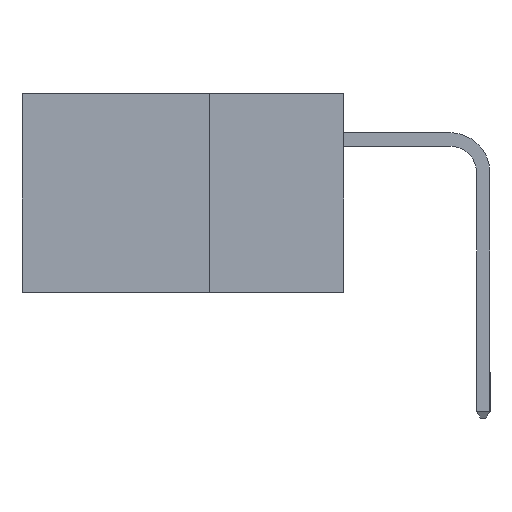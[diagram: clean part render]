
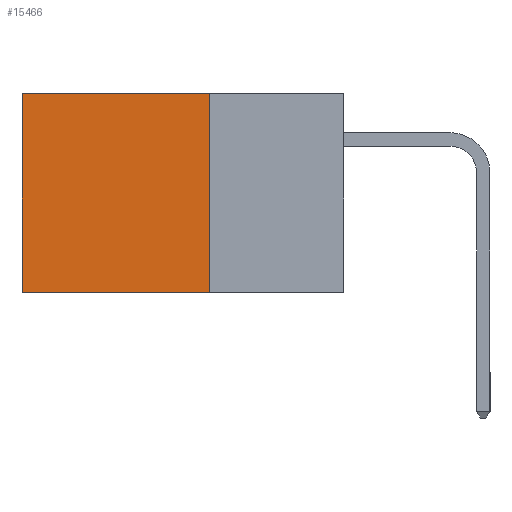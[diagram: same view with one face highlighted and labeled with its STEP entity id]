
A CAD part, left-side view. The second image highlights one B-rep face of the part: STEP entity #15466.
In plain terms, the highlighted planar face has unit normal (-1, 0, 0).
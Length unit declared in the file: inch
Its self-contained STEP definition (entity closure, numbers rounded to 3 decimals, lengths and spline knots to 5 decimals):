
#284 = DIRECTION ( 'NONE',  ( 1., 0., 0. ) ) ;
#853 = DIRECTION ( 'NONE',  ( 0., 1., 0. ) ) ;
#2207 = CARTESIAN_POINT ( 'NONE',  ( 0.2615, 0.6, -0.37 ) ) ;
#4711 = CARTESIAN_POINT ( 'NONE',  ( 0.2615, 0.25, -0.37 ) ) ;
#6311 = LINE ( 'NONE', #13989, #12401 ) ;
#6320 = CARTESIAN_POINT ( 'NONE',  ( 0.2615, 0.6, 0. ) ) ;
#6404 = AXIS2_PLACEMENT_3D ( 'NONE', #8105, #284, #21174 ) ;
#6442 = DIRECTION ( 'NONE',  ( 0., 0., -1. ) ) ;
#6992 = VERTEX_POINT ( 'NONE', #2207 ) ;
#7033 = EDGE_CURVE ( 'NONE', #23783, #6992, #16089, .T. ) ;
#7888 = CARTESIAN_POINT ( 'NONE',  ( 0.2615, 0.25, 0. ) ) ;
#7927 = VECTOR ( 'NONE', #9614, 39.37008 ) ;
#8105 = CARTESIAN_POINT ( 'NONE',  ( 0.2615, 0.25, -0.37 ) ) ;
#8793 = ORIENTED_EDGE ( 'NONE', *, *, #12808, .T. ) ;
#9614 = DIRECTION ( 'NONE',  ( 0., 0., -1. ) ) ;
#10585 = CARTESIAN_POINT ( 'NONE',  ( 0.2615, 0.25, -0.37 ) ) ;
#11609 = EDGE_CURVE ( 'NONE', #22007, #23783, #20937, .T. ) ;
#11728 = ORIENTED_EDGE ( 'NONE', *, *, #7033, .F. ) ;
#12401 = VECTOR ( 'NONE', #853, 39.37008 ) ;
#12678 = VERTEX_POINT ( 'NONE', #6320 ) ;
#12743 = VECTOR ( 'NONE', #19957, 39.37008 ) ;
#12808 = EDGE_CURVE ( 'NONE', #12678, #6992, #19885, .T. ) ;
#13989 = CARTESIAN_POINT ( 'NONE',  ( 0.2615, 0.25, 0. ) ) ;
#14927 = ORIENTED_EDGE ( 'NONE', *, *, #11609, .F. ) ;
#15466 = ADVANCED_FACE ( 'NONE', ( #17565 ), #15564, .F. ) ;
#15564 = PLANE ( 'NONE',  #6404 ) ;
#15610 = ORIENTED_EDGE ( 'NONE', *, *, #17685, .T. ) ;
#16089 = LINE ( 'NONE', #10585, #12743 ) ;
#16621 = VECTOR ( 'NONE', #6442, 39.37008 ) ;
#16666 = EDGE_LOOP ( 'NONE', ( #8793, #11728, #14927, #15610 ) ) ;
#17565 = FACE_OUTER_BOUND ( 'NONE', #16666, .T. ) ;
#17685 = EDGE_CURVE ( 'NONE', #22007, #12678, #6311, .T. ) ;
#17890 = CARTESIAN_POINT ( 'NONE',  ( 0.2615, 0.6, -0.37 ) ) ;
#19885 = LINE ( 'NONE', #17890, #16621 ) ;
#19957 = DIRECTION ( 'NONE',  ( 0., 1., 0. ) ) ;
#20937 = LINE ( 'NONE', #24289, #7927 ) ;
#21174 = DIRECTION ( 'NONE',  ( 0., 0., -1. ) ) ;
#22007 = VERTEX_POINT ( 'NONE', #7888 ) ;
#23783 = VERTEX_POINT ( 'NONE', #4711 ) ;
#24289 = CARTESIAN_POINT ( 'NONE',  ( 0.2615, 0.25, -0.37 ) ) ;
